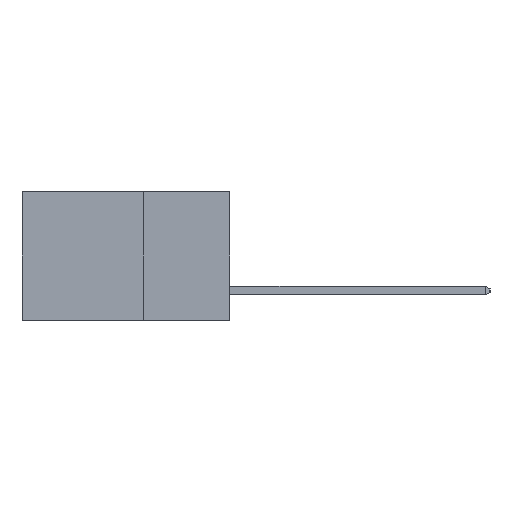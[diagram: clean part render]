
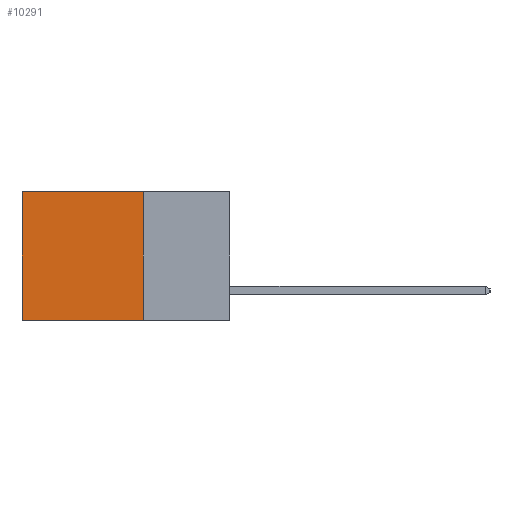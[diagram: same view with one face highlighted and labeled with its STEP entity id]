
A CAD part, left-side view. The second image highlights one B-rep face of the part: STEP entity #10291.
In plain terms, the highlighted planar face has unit normal (-1, 0, 0).
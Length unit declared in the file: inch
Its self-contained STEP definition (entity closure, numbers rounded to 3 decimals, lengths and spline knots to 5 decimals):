
#80 = EDGE_LOOP ( 'NONE', ( #4027, #10360, #2511, #13503 ) ) ;
#698 = CARTESIAN_POINT ( 'NONE',  ( 0.298, 0.25, 0. ) ) ;
#1560 = VECTOR ( 'NONE', #9802, 39.37008 ) ;
#2172 = DIRECTION ( 'NONE',  ( 0., 0., -1. ) ) ;
#2184 = CARTESIAN_POINT ( 'NONE',  ( 0.298, 0.25, 0. ) ) ;
#2511 = ORIENTED_EDGE ( 'NONE', *, *, #16435, .F. ) ;
#3128 = VECTOR ( 'NONE', #4269, 39.37008 ) ;
#3793 = AXIS2_PLACEMENT_3D ( 'NONE', #698, #10374, #2172 ) ;
#4027 = ORIENTED_EDGE ( 'NONE', *, *, #12010, .T. ) ;
#4269 = DIRECTION ( 'NONE',  ( 0., 1., 0. ) ) ;
#4743 = CARTESIAN_POINT ( 'NONE',  ( 0.298, 0.25, 0. ) ) ;
#4838 = CARTESIAN_POINT ( 'NONE',  ( 0.298, 0.6, 0. ) ) ;
#5416 = VERTEX_POINT ( 'NONE', #4743 ) ;
#5496 = VERTEX_POINT ( 'NONE', #15633 ) ;
#5860 = CARTESIAN_POINT ( 'NONE',  ( 0.298, 0.6, 0. ) ) ;
#8388 = EDGE_CURVE ( 'NONE', #5416, #10286, #17185, .T. ) ;
#8714 = VECTOR ( 'NONE', #16419, 39.37008 ) ;
#9042 = PLANE ( 'NONE',  #3793 ) ;
#9406 = VECTOR ( 'NONE', #13072, 39.37008 ) ;
#9802 = DIRECTION ( 'NONE',  ( 0., 0., -1. ) ) ;
#10286 = VERTEX_POINT ( 'NONE', #4838 ) ;
#10291 = ADVANCED_FACE ( 'NONE', ( #15917 ), #9042, .F. ) ;
#10360 = ORIENTED_EDGE ( 'NONE', *, *, #10612, .F. ) ;
#10374 = DIRECTION ( 'NONE',  ( 1., 0., 0. ) ) ;
#10612 = EDGE_CURVE ( 'NONE', #12963, #5496, #13944, .T. ) ;
#11956 = CARTESIAN_POINT ( 'NONE',  ( 0.298, 0.25, -0.37 ) ) ;
#12010 = EDGE_CURVE ( 'NONE', #10286, #5496, #16107, .T. ) ;
#12418 = CARTESIAN_POINT ( 'NONE',  ( 0.298, 0.25, 0. ) ) ;
#12459 = LINE ( 'NONE', #12418, #1560 ) ;
#12963 = VERTEX_POINT ( 'NONE', #14466 ) ;
#13072 = DIRECTION ( 'NONE',  ( 0., 1., 0. ) ) ;
#13503 = ORIENTED_EDGE ( 'NONE', *, *, #8388, .T. ) ;
#13944 = LINE ( 'NONE', #11956, #3128 ) ;
#14466 = CARTESIAN_POINT ( 'NONE',  ( 0.298, 0.25, -0.37 ) ) ;
#15633 = CARTESIAN_POINT ( 'NONE',  ( 0.298, 0.6, -0.37 ) ) ;
#15917 = FACE_OUTER_BOUND ( 'NONE', #80, .T. ) ;
#16107 = LINE ( 'NONE', #5860, #8714 ) ;
#16419 = DIRECTION ( 'NONE',  ( 0., 0., -1. ) ) ;
#16435 = EDGE_CURVE ( 'NONE', #5416, #12963, #12459, .T. ) ;
#17185 = LINE ( 'NONE', #2184, #9406 ) ;
